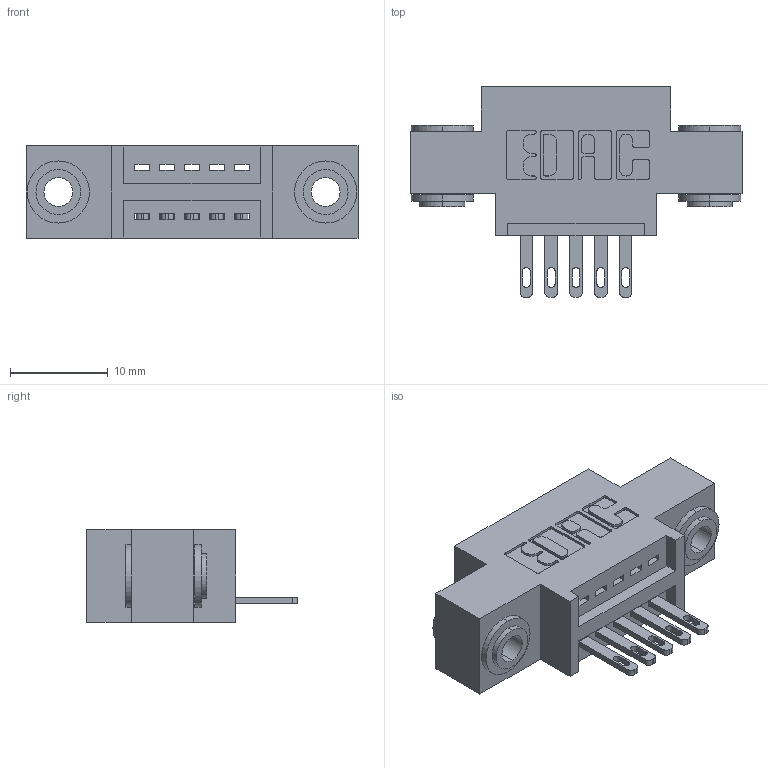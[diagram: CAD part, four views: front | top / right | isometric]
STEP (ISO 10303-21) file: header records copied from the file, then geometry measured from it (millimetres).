
FILE_DESCRIPTION (( 'STEP AP203' ), '1' );
FILE_NAME ('895-005-500-603.STEP', '2020-09-24T21:29:04', ( '' ), ( '' ), 'SwSTEP 2.0', 'SolidWorks 2020', '' );
FILE_SCHEMA (( 'CONFIG_CONTROL_DESIGN' ));
Length unit declared in the file: inch
Products named in the file (4): 845 Part_0.170 Offset - 0.156 Dia-TH; 345-250-002_345-250-002-102; 895-005-500-603; 345-292-001_345-293-100
Assembly tree (8 placements, depth 2):
  895-005-500-603
    845 Part_0.170 Offset - 0.156 Dia-TH
    345-292-001_345-293-100  x5
    345-250-002_345-250-002-102  x2
Bounding box: 33.91 x 21.51 x 9.4 mm (x, y, z)
Volume: 2826.7 mm3; surface area: 3605.9 mm2
Topology: 8 solids, 8 shells, 438 faces, 1269 edges, 842 vertices
Faces by surface type: plane 264, cylinder 166, cone 8
Entity records: 9456 total; most frequent: CARTESIAN_POINT 1618, ORIENTED_EDGE 1550, DIRECTION 1499, EDGE_CURVE 775, VECTOR 595, LINE 595, VERTEX_POINT 514, AXIS2_PLACEMENT_3D 452
